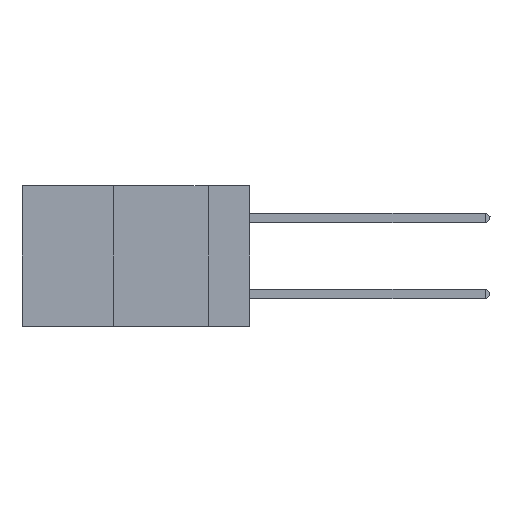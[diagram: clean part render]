
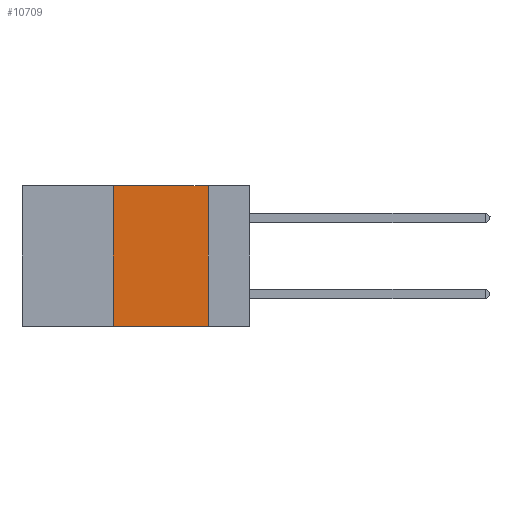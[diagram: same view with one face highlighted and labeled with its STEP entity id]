
A CAD part, left-side view. The second image highlights one B-rep face of the part: STEP entity #10709.
In plain terms, the highlighted planar face has unit normal (-1, 0, 0).
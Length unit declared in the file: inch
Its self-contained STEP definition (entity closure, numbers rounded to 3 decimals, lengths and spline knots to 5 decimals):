
#499 = LINE ( 'NONE', #5292, #11329 ) ;
#777 = DIRECTION ( 'NONE',  ( 1., 0., 0. ) ) ;
#1087 = EDGE_CURVE ( 'NONE', #1201, #5428, #6162, .T. ) ;
#1201 = VERTEX_POINT ( 'NONE', #12273 ) ;
#2155 = DIRECTION ( 'NONE',  ( 0., -1., 0. ) ) ;
#2236 = VERTEX_POINT ( 'NONE', #9572 ) ;
#2239 = CARTESIAN_POINT ( 'NONE',  ( 0., 0.36, 0. ) ) ;
#3301 = DIRECTION ( 'NONE',  ( 0., -1., 0. ) ) ;
#3313 = DIRECTION ( 'NONE',  ( 0., 0., 1. ) ) ;
#3401 = VECTOR ( 'NONE', #3313, 39.37008 ) ;
#3754 = CARTESIAN_POINT ( 'NONE',  ( 0., 0.11, -0.37 ) ) ;
#3836 = CARTESIAN_POINT ( 'NONE',  ( 0., 0.11, 0. ) ) ;
#5007 = ORIENTED_EDGE ( 'NONE', *, *, #9726, .F. ) ;
#5292 = CARTESIAN_POINT ( 'NONE',  ( 0., 0.6, 0. ) ) ;
#5302 = CARTESIAN_POINT ( 'NONE',  ( 0., 0.11, 0. ) ) ;
#5428 = VERTEX_POINT ( 'NONE', #3754 ) ;
#5526 = LINE ( 'NONE', #5302, #13496 ) ;
#5578 = DIRECTION ( 'NONE',  ( 0., 0., -1. ) ) ;
#5849 = VECTOR ( 'NONE', #3301, 39.37008 ) ;
#6162 = LINE ( 'NONE', #6172, #5849 ) ;
#6172 = CARTESIAN_POINT ( 'NONE',  ( 0., 0.6, -0.37 ) ) ;
#7389 = EDGE_CURVE ( 'NONE', #12790, #5428, #5526, .T. ) ;
#7397 = AXIS2_PLACEMENT_3D ( 'NONE', #9176, #777, #8169 ) ;
#8169 = DIRECTION ( 'NONE',  ( 0., 0., -1. ) ) ;
#8447 = EDGE_CURVE ( 'NONE', #1201, #2236, #11724, .T. ) ;
#9113 = EDGE_LOOP ( 'NONE', ( #12826, #5007, #10337, #9895 ) ) ;
#9176 = CARTESIAN_POINT ( 'NONE',  ( 0., 0.6, 0. ) ) ;
#9572 = CARTESIAN_POINT ( 'NONE',  ( 0., 0.36, 0. ) ) ;
#9726 = EDGE_CURVE ( 'NONE', #2236, #12790, #499, .T. ) ;
#9895 = ORIENTED_EDGE ( 'NONE', *, *, #1087, .T. ) ;
#10337 = ORIENTED_EDGE ( 'NONE', *, *, #8447, .F. ) ;
#10709 = ADVANCED_FACE ( 'NONE', ( #13112 ), #11256, .F. ) ;
#11256 = PLANE ( 'NONE',  #7397 ) ;
#11329 = VECTOR ( 'NONE', #2155, 39.37008 ) ;
#11724 = LINE ( 'NONE', #2239, #3401 ) ;
#12273 = CARTESIAN_POINT ( 'NONE',  ( 0., 0.36, -0.37 ) ) ;
#12790 = VERTEX_POINT ( 'NONE', #3836 ) ;
#12826 = ORIENTED_EDGE ( 'NONE', *, *, #7389, .F. ) ;
#13112 = FACE_OUTER_BOUND ( 'NONE', #9113, .T. ) ;
#13496 = VECTOR ( 'NONE', #5578, 39.37008 ) ;
